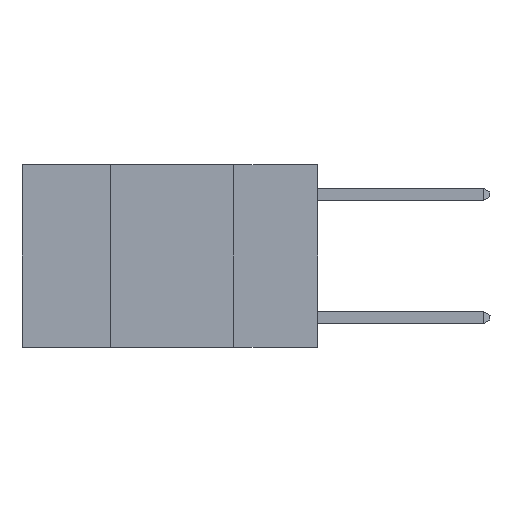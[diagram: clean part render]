
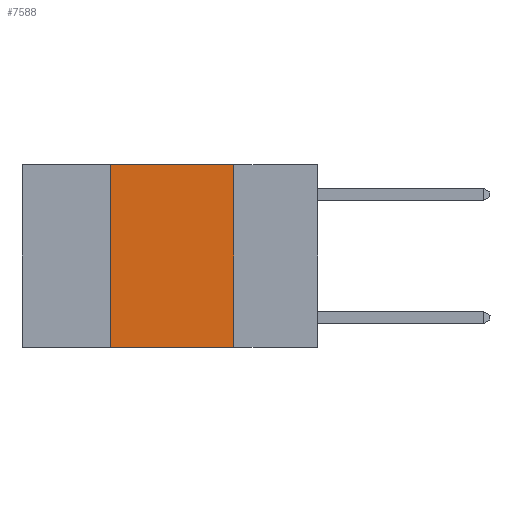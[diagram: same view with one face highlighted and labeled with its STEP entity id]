
A CAD part, left-side view. The second image highlights one B-rep face of the part: STEP entity #7588.
In plain terms, the highlighted planar face has unit normal (-1, 0, 0).
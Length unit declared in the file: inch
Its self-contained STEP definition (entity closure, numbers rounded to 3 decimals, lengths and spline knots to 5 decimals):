
#189 = LINE ( 'NONE', #6834, #2314 ) ;
#194 = EDGE_CURVE ( 'NONE', #4618, #2072, #5531, .T. ) ;
#201 = ORIENTED_EDGE ( 'NONE', *, *, #194, .F. ) ;
#732 = ORIENTED_EDGE ( 'NONE', *, *, #1415, .T. ) ;
#818 = EDGE_CURVE ( 'NONE', #6299, #5563, #4005, .T. ) ;
#1415 = EDGE_CURVE ( 'NONE', #6299, #2072, #5930, .T. ) ;
#1853 = VECTOR ( 'NONE', #6225, 39.37008 ) ;
#1865 = CARTESIAN_POINT ( 'NONE',  ( 0., 0.6, -0.37 ) ) ;
#2024 = CARTESIAN_POINT ( 'NONE',  ( 0., 0.6, 0. ) ) ;
#2072 = VERTEX_POINT ( 'NONE', #5330 ) ;
#2156 = VECTOR ( 'NONE', #2529, 39.37008 ) ;
#2314 = VECTOR ( 'NONE', #2680, 39.37008 ) ;
#2481 = AXIS2_PLACEMENT_3D ( 'NONE', #2024, #7609, #3527 ) ;
#2529 = DIRECTION ( 'NONE',  ( 0., -1., 0. ) ) ;
#2680 = DIRECTION ( 'NONE',  ( 0., -1., 0. ) ) ;
#3084 = DIRECTION ( 'NONE',  ( 0., 0., -1. ) ) ;
#3452 = VECTOR ( 'NONE', #3084, 39.37008 ) ;
#3527 = DIRECTION ( 'NONE',  ( 0., 0., -1. ) ) ;
#3799 = CARTESIAN_POINT ( 'NONE',  ( 0., 0.17, 0. ) ) ;
#4005 = LINE ( 'NONE', #8196, #1853 ) ;
#4618 = VERTEX_POINT ( 'NONE', #8683 ) ;
#4811 = EDGE_LOOP ( 'NONE', ( #201, #6748, #7868, #732 ) ) ;
#5330 = CARTESIAN_POINT ( 'NONE',  ( 0., 0.17, -0.37 ) ) ;
#5531 = LINE ( 'NONE', #3799, #3452 ) ;
#5563 = VERTEX_POINT ( 'NONE', #7022 ) ;
#5594 = PLANE ( 'NONE',  #2481 ) ;
#5930 = LINE ( 'NONE', #1865, #2156 ) ;
#6225 = DIRECTION ( 'NONE',  ( 0., 0., 1. ) ) ;
#6299 = VERTEX_POINT ( 'NONE', #7394 ) ;
#6748 = ORIENTED_EDGE ( 'NONE', *, *, #7487, .F. ) ;
#6807 = FACE_OUTER_BOUND ( 'NONE', #4811, .T. ) ;
#6834 = CARTESIAN_POINT ( 'NONE',  ( 0., 0.6, 0. ) ) ;
#7022 = CARTESIAN_POINT ( 'NONE',  ( 0., 0.42, 0. ) ) ;
#7394 = CARTESIAN_POINT ( 'NONE',  ( 0., 0.42, -0.37 ) ) ;
#7487 = EDGE_CURVE ( 'NONE', #5563, #4618, #189, .T. ) ;
#7588 = ADVANCED_FACE ( 'NONE', ( #6807 ), #5594, .F. ) ;
#7609 = DIRECTION ( 'NONE',  ( 1., 0., 0. ) ) ;
#7868 = ORIENTED_EDGE ( 'NONE', *, *, #818, .F. ) ;
#8196 = CARTESIAN_POINT ( 'NONE',  ( 0., 0.42, 0. ) ) ;
#8683 = CARTESIAN_POINT ( 'NONE',  ( 0., 0.17, 0. ) ) ;
